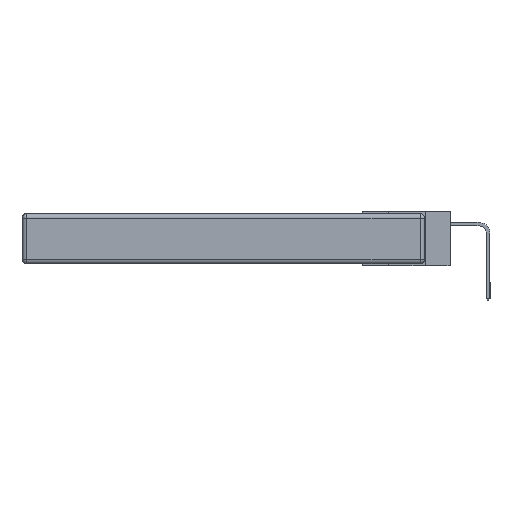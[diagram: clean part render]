
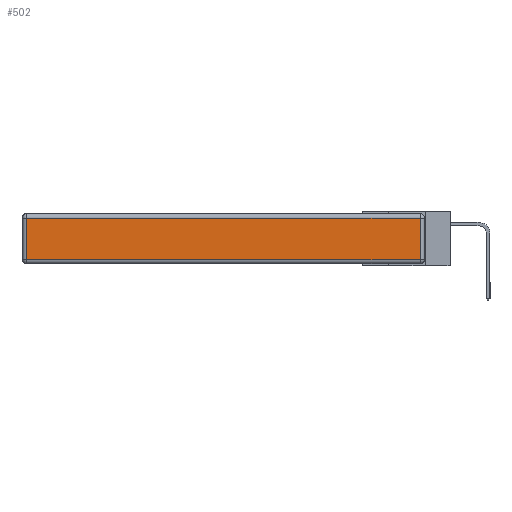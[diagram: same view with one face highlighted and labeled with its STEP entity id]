
A CAD part, left-side view. The second image highlights one B-rep face of the part: STEP entity #502.
In plain terms, the highlighted planar face has unit normal (-1, 0, 0).
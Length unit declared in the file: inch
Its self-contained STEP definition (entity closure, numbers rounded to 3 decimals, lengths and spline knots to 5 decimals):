
#427 = EDGE_LOOP ( 'NONE', ( #3411, #3269, #11883, #10361 ) ) ;
#502 = ADVANCED_FACE ( 'NONE', ( #5885 ), #9320, .T. ) ;
#2187 = CARTESIAN_POINT ( 'NONE',  ( 0., 0., -0.343 ) ) ;
#3269 = ORIENTED_EDGE ( 'NONE', *, *, #15141, .T. ) ;
#3411 = ORIENTED_EDGE ( 'NONE', *, *, #6564, .T. ) ;
#4249 = EDGE_CURVE ( 'NONE', #17393, #17798, #5071, .T. ) ;
#4634 = VECTOR ( 'NONE', #16330, 39.37008 ) ;
#4846 = EDGE_CURVE ( 'NONE', #17798, #17536, #17978, .T. ) ;
#4880 = CARTESIAN_POINT ( 'NONE',  ( 0., 0., -0.313 ) ) ;
#5071 = LINE ( 'NONE', #14143, #6210 ) ;
#5885 = FACE_OUTER_BOUND ( 'NONE', #427, .T. ) ;
#6210 = VECTOR ( 'NONE', #6923, 39.37008 ) ;
#6564 = EDGE_CURVE ( 'NONE', #17536, #9442, #8011, .T. ) ;
#6643 = AXIS2_PLACEMENT_3D ( 'NONE', #2187, #7727, #9431 ) ;
#6923 = DIRECTION ( 'NONE',  ( 0., 1., 0. ) ) ;
#7727 = DIRECTION ( 'NONE',  ( -1., 0., 0. ) ) ;
#7753 = VECTOR ( 'NONE', #10675, 39.37008 ) ;
#7789 = VECTOR ( 'NONE', #16563, 39.37008 ) ;
#8011 = LINE ( 'NONE', #4880, #7789 ) ;
#8786 = CARTESIAN_POINT ( 'NONE',  ( 0., 0.03, -0.03 ) ) ;
#8825 = CARTESIAN_POINT ( 'NONE',  ( 0., 0.03, -0.343 ) ) ;
#9320 = PLANE ( 'NONE',  #6643 ) ;
#9431 = DIRECTION ( 'NONE',  ( 0., 0., 1. ) ) ;
#9442 = VERTEX_POINT ( 'NONE', #17721 ) ;
#10361 = ORIENTED_EDGE ( 'NONE', *, *, #4846, .T. ) ;
#10369 = CARTESIAN_POINT ( 'NONE',  ( 0., 2.72, -0.313 ) ) ;
#10675 = DIRECTION ( 'NONE',  ( 0., 0., -1. ) ) ;
#11883 = ORIENTED_EDGE ( 'NONE', *, *, #4249, .T. ) ;
#14143 = CARTESIAN_POINT ( 'NONE',  ( 0., 2.75, -0.03 ) ) ;
#15004 = CARTESIAN_POINT ( 'NONE',  ( 0., 2.72, -0.343 ) ) ;
#15141 = EDGE_CURVE ( 'NONE', #9442, #17393, #15336, .T. ) ;
#15336 = LINE ( 'NONE', #8825, #4634 ) ;
#15411 = CARTESIAN_POINT ( 'NONE',  ( 0., 2.72, -0.03 ) ) ;
#16330 = DIRECTION ( 'NONE',  ( 0., 0., 1. ) ) ;
#16563 = DIRECTION ( 'NONE',  ( 0., -1., 0. ) ) ;
#17393 = VERTEX_POINT ( 'NONE', #8786 ) ;
#17536 = VERTEX_POINT ( 'NONE', #10369 ) ;
#17721 = CARTESIAN_POINT ( 'NONE',  ( 0., 0.03, -0.313 ) ) ;
#17798 = VERTEX_POINT ( 'NONE', #15411 ) ;
#17978 = LINE ( 'NONE', #15004, #7753 ) ;
